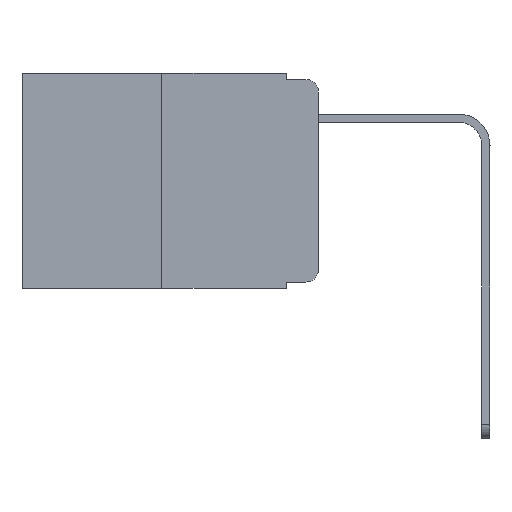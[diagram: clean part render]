
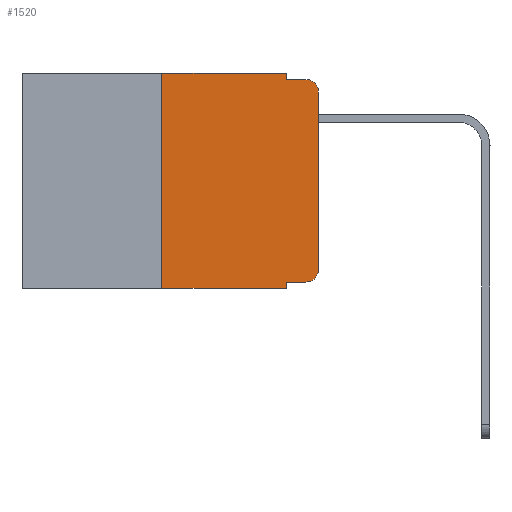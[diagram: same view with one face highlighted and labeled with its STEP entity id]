
A CAD part, left-side view. The second image highlights one B-rep face of the part: STEP entity #1520.
In plain terms, the highlighted planar face has unit normal (-1, 0, 0).
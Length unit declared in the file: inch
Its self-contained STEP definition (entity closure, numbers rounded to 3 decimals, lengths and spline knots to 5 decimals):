
#241 = DIRECTION ( 'NONE',  ( 0., 0., -1. ) ) ;
#275 = CARTESIAN_POINT ( 'NONE',  ( 0., 0., -0.313 ) ) ;
#674 = EDGE_CURVE ( 'NONE', #11844, #17401, #7318, .T. ) ;
#867 = VERTEX_POINT ( 'NONE', #7323 ) ;
#872 = ORIENTED_EDGE ( 'NONE', *, *, #4438, .F. ) ;
#1520 = ADVANCED_FACE ( 'NONE', ( #13691 ), #6329, .F. ) ;
#1636 = VERTEX_POINT ( 'NONE', #10823 ) ;
#1712 = DIRECTION ( 'NONE',  ( 0., 0., -1. ) ) ;
#1737 = CARTESIAN_POINT ( 'NONE',  ( 0., 0.051, -0.333 ) ) ;
#1795 = CARTESIAN_POINT ( 'NONE',  ( 0., 0.051, 0. ) ) ;
#1846 = DIRECTION ( 'NONE',  ( 0., 0., -1. ) ) ;
#2021 = CIRCLE ( 'NONE', #8757, 0.02 ) ;
#2114 = CARTESIAN_POINT ( 'NONE',  ( 0., 0.02, -0.313 ) ) ;
#2277 = VERTEX_POINT ( 'NONE', #11321 ) ;
#2700 = CARTESIAN_POINT ( 'NONE',  ( 0., 0.051, -0.333 ) ) ;
#2933 = CARTESIAN_POINT ( 'NONE',  ( 0., 0.051, 0. ) ) ;
#3035 = EDGE_CURVE ( 'NONE', #867, #2277, #9380, .T. ) ;
#3083 = DIRECTION ( 'NONE',  ( 0., -1., 0. ) ) ;
#3977 = LINE ( 'NONE', #15293, #10192 ) ;
#4418 = VERTEX_POINT ( 'NONE', #9122 ) ;
#4438 = EDGE_CURVE ( 'NONE', #2277, #6936, #5549, .T. ) ;
#4573 = EDGE_CURVE ( 'NONE', #1636, #5825, #6194, .T. ) ;
#4740 = VERTEX_POINT ( 'NONE', #275 ) ;
#5150 = CARTESIAN_POINT ( 'NONE',  ( 0., 0.473, 0. ) ) ;
#5380 = EDGE_CURVE ( 'NONE', #4740, #4418, #10223, .T. ) ;
#5480 = CARTESIAN_POINT ( 'NONE',  ( 0., 0.473, 0. ) ) ;
#5549 = LINE ( 'NONE', #5150, #14102 ) ;
#5825 = VERTEX_POINT ( 'NONE', #12566 ) ;
#5995 = EDGE_CURVE ( 'NONE', #17401, #4740, #2021, .T. ) ;
#6194 = LINE ( 'NONE', #16208, #10049 ) ;
#6329 = PLANE ( 'NONE',  #11193 ) ;
#6936 = VERTEX_POINT ( 'NONE', #2933 ) ;
#7143 = ORIENTED_EDGE ( 'NONE', *, *, #12339, .F. ) ;
#7318 = LINE ( 'NONE', #2700, #9239 ) ;
#7323 = CARTESIAN_POINT ( 'NONE',  ( 0., 0.25, -0.343 ) ) ;
#7500 = VECTOR ( 'NONE', #241, 39.37008 ) ;
#7924 = DIRECTION ( 'NONE',  ( 0., -1., 0. ) ) ;
#8451 = ORIENTED_EDGE ( 'NONE', *, *, #10126, .F. ) ;
#8506 = EDGE_CURVE ( 'NONE', #4418, #5825, #15434, .T. ) ;
#8525 = VECTOR ( 'NONE', #13036, 39.37008 ) ;
#8721 = DIRECTION ( 'NONE',  ( -1., 0., 0. ) ) ;
#8757 = AXIS2_PLACEMENT_3D ( 'NONE', #2114, #14464, #15728 ) ;
#9122 = CARTESIAN_POINT ( 'NONE',  ( 0., 0., -0.03 ) ) ;
#9239 = VECTOR ( 'NONE', #16414, 39.37008 ) ;
#9380 = LINE ( 'NONE', #10295, #8525 ) ;
#9413 = DIRECTION ( 'NONE',  ( 0., -1., 0. ) ) ;
#9592 = ORIENTED_EDGE ( 'NONE', *, *, #5380, .T. ) ;
#9610 = DIRECTION ( 'NONE',  ( 1., 0., 0. ) ) ;
#10049 = VECTOR ( 'NONE', #9413, 39.37008 ) ;
#10126 = EDGE_CURVE ( 'NONE', #11844, #12321, #17101, .T. ) ;
#10192 = VECTOR ( 'NONE', #3083, 39.37008 ) ;
#10223 = LINE ( 'NONE', #17064, #11694 ) ;
#10295 = CARTESIAN_POINT ( 'NONE',  ( 0., 0.25, 0. ) ) ;
#10823 = CARTESIAN_POINT ( 'NONE',  ( 0., 0.051, -0.01 ) ) ;
#11145 = CARTESIAN_POINT ( 'NONE',  ( 0., 0.051, -0.343 ) ) ;
#11193 = AXIS2_PLACEMENT_3D ( 'NONE', #5480, #9610, #16407 ) ;
#11222 = ORIENTED_EDGE ( 'NONE', *, *, #4573, .F. ) ;
#11280 = ORIENTED_EDGE ( 'NONE', *, *, #674, .T. ) ;
#11321 = CARTESIAN_POINT ( 'NONE',  ( 0., 0.25, 0. ) ) ;
#11694 = VECTOR ( 'NONE', #15805, 39.37008 ) ;
#11844 = VERTEX_POINT ( 'NONE', #1737 ) ;
#12321 = VERTEX_POINT ( 'NONE', #11145 ) ;
#12339 = EDGE_CURVE ( 'NONE', #6936, #1636, #16636, .T. ) ;
#12566 = CARTESIAN_POINT ( 'NONE',  ( 0., 0.02, -0.01 ) ) ;
#13036 = DIRECTION ( 'NONE',  ( 0., 0., 1. ) ) ;
#13043 = ORIENTED_EDGE ( 'NONE', *, *, #8506, .T. ) ;
#13103 = EDGE_CURVE ( 'NONE', #867, #12321, #3977, .T. ) ;
#13112 = EDGE_LOOP ( 'NONE', ( #9592, #13043, #11222, #7143, #872, #17017, #14183, #8451, #11280, #14294 ) ) ;
#13360 = AXIS2_PLACEMENT_3D ( 'NONE', #16898, #8721, #1846 ) ;
#13691 = FACE_OUTER_BOUND ( 'NONE', #13112, .T. ) ;
#13775 = CARTESIAN_POINT ( 'NONE',  ( 0., 0.051, 0. ) ) ;
#14102 = VECTOR ( 'NONE', #7924, 39.37008 ) ;
#14183 = ORIENTED_EDGE ( 'NONE', *, *, #13103, .T. ) ;
#14294 = ORIENTED_EDGE ( 'NONE', *, *, #5995, .T. ) ;
#14464 = DIRECTION ( 'NONE',  ( -1., 0., 0. ) ) ;
#15293 = CARTESIAN_POINT ( 'NONE',  ( 0., 0.473, -0.343 ) ) ;
#15434 = CIRCLE ( 'NONE', #13360, 0.02 ) ;
#15728 = DIRECTION ( 'NONE',  ( 0., 0., -1. ) ) ;
#15805 = DIRECTION ( 'NONE',  ( 0., 0., 1. ) ) ;
#16208 = CARTESIAN_POINT ( 'NONE',  ( 0., 0.051, -0.01 ) ) ;
#16407 = DIRECTION ( 'NONE',  ( 0., 0., -1. ) ) ;
#16414 = DIRECTION ( 'NONE',  ( 0., -1., 0. ) ) ;
#16636 = LINE ( 'NONE', #13775, #17057 ) ;
#16898 = CARTESIAN_POINT ( 'NONE',  ( 0., 0.02, -0.03 ) ) ;
#17017 = ORIENTED_EDGE ( 'NONE', *, *, #3035, .F. ) ;
#17057 = VECTOR ( 'NONE', #1712, 39.37008 ) ;
#17064 = CARTESIAN_POINT ( 'NONE',  ( 0., 0., 0. ) ) ;
#17101 = LINE ( 'NONE', #1795, #7500 ) ;
#17224 = CARTESIAN_POINT ( 'NONE',  ( 0., 0.02, -0.333 ) ) ;
#17401 = VERTEX_POINT ( 'NONE', #17224 ) ;
